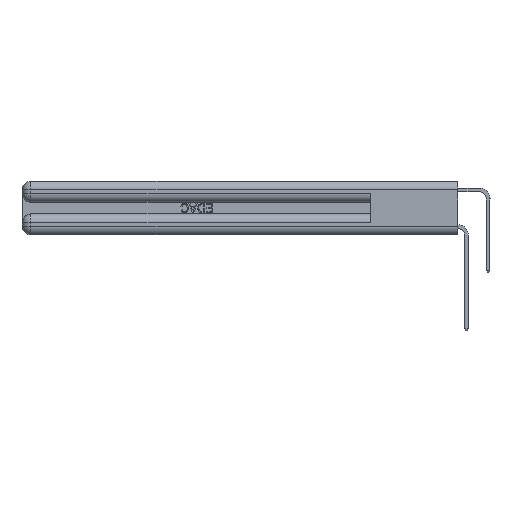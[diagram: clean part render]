
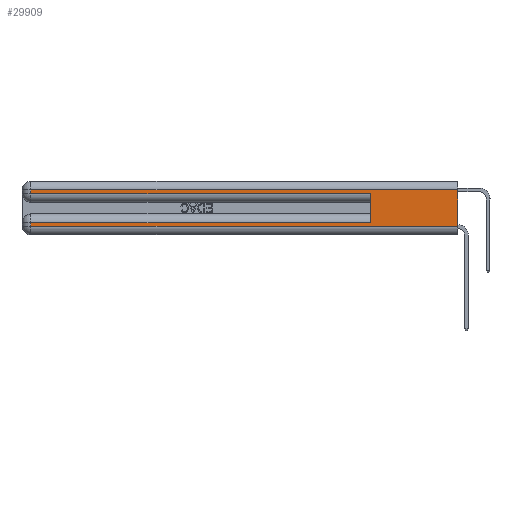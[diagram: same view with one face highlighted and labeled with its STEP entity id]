
A CAD part, left-side view. The second image highlights one B-rep face of the part: STEP entity #29909.
In plain terms, the highlighted planar face has unit normal (-1, 0, 0).
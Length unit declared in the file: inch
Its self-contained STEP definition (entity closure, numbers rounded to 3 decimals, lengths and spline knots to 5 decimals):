
#688 = CARTESIAN_POINT ( 'NONE',  ( 0., 0., 0.31 ) ) ;
#2216 = DIRECTION ( 'NONE',  ( 0., 0., -1. ) ) ;
#2385 = CARTESIAN_POINT ( 'NONE',  ( 0., 0.6, 0.285 ) ) ;
#2524 = EDGE_CURVE ( 'NONE', #15387, #31650, #4604, .T. ) ;
#3878 = CARTESIAN_POINT ( 'NONE',  ( 0., 0., 0.06 ) ) ;
#4311 = FACE_OUTER_BOUND ( 'NONE', #28286, .T. ) ;
#4604 = LINE ( 'NONE', #30196, #15029 ) ;
#4754 = DIRECTION ( 'NONE',  ( 1., 0., 0. ) ) ;
#4879 = CARTESIAN_POINT ( 'NONE',  ( 0., 0., 0.085 ) ) ;
#4961 = CARTESIAN_POINT ( 'NONE',  ( 0., 0.6, 0.145 ) ) ;
#4972 = DIRECTION ( 'NONE',  ( 0., -1., 0. ) ) ;
#5525 = LINE ( 'NONE', #33076, #29310 ) ;
#6470 = LINE ( 'NONE', #688, #27855 ) ;
#6865 = LINE ( 'NONE', #4879, #18047 ) ;
#7455 = DIRECTION ( 'NONE',  ( 0., 0., -1. ) ) ;
#8250 = EDGE_CURVE ( 'NONE', #22553, #27764, #6470, .T. ) ;
#8692 = VERTEX_POINT ( 'NONE', #15532 ) ;
#9332 = ORIENTED_EDGE ( 'NONE', *, *, #22059, .T. ) ;
#9527 = VECTOR ( 'NONE', #7455, 39.37008 ) ;
#10952 = ORIENTED_EDGE ( 'NONE', *, *, #20785, .F. ) ;
#11116 = LINE ( 'NONE', #4961, #17175 ) ;
#11144 = CARTESIAN_POINT ( 'NONE',  ( 0., 2.94, 0.31 ) ) ;
#13689 = CARTESIAN_POINT ( 'NONE',  ( 0., 2.94, 0.285 ) ) ;
#13787 = CARTESIAN_POINT ( 'NONE',  ( 0., 0., 0.06 ) ) ;
#13980 = CARTESIAN_POINT ( 'NONE',  ( 0., 0., 0.37 ) ) ;
#14259 = VERTEX_POINT ( 'NONE', #28304 ) ;
#14722 = LINE ( 'NONE', #20456, #9527 ) ;
#15029 = VECTOR ( 'NONE', #4972, 39.37008 ) ;
#15387 = VERTEX_POINT ( 'NONE', #13689 ) ;
#15532 = CARTESIAN_POINT ( 'NONE',  ( 0., 2.94, 0.06 ) ) ;
#16573 = LINE ( 'NONE', #13787, #28685 ) ;
#17175 = VECTOR ( 'NONE', #18098, 39.37008 ) ;
#17604 = ORIENTED_EDGE ( 'NONE', *, *, #8250, .T. ) ;
#17777 = CARTESIAN_POINT ( 'NONE',  ( 0., 0., 0.37 ) ) ;
#18047 = VECTOR ( 'NONE', #20168, 39.37008 ) ;
#18098 = DIRECTION ( 'NONE',  ( 0., 0., 1. ) ) ;
#18941 = DIRECTION ( 'NONE',  ( 0., 0., -1. ) ) ;
#19156 = CARTESIAN_POINT ( 'NONE',  ( 0., 0., 0.31 ) ) ;
#19185 = VERTEX_POINT ( 'NONE', #3878 ) ;
#19994 = AXIS2_PLACEMENT_3D ( 'NONE', #17777, #4754, #30559 ) ;
#20168 = DIRECTION ( 'NONE',  ( 0., 1., 0. ) ) ;
#20456 = CARTESIAN_POINT ( 'NONE',  ( 0., 2.94, 0.37 ) ) ;
#20785 = EDGE_CURVE ( 'NONE', #22553, #19185, #29424, .T. ) ;
#20949 = DIRECTION ( 'NONE',  ( 0., 1., 0. ) ) ;
#22059 = EDGE_CURVE ( 'NONE', #28037, #14259, #6865, .T. ) ;
#22553 = VERTEX_POINT ( 'NONE', #19156 ) ;
#23087 = PLANE ( 'NONE',  #19994 ) ;
#23167 = ORIENTED_EDGE ( 'NONE', *, *, #28883, .T. ) ;
#24087 = EDGE_CURVE ( 'NONE', #27764, #15387, #14722, .T. ) ;
#24133 = EDGE_CURVE ( 'NONE', #28037, #31650, #11116, .T. ) ;
#24204 = ORIENTED_EDGE ( 'NONE', *, *, #2524, .T. ) ;
#25109 = ORIENTED_EDGE ( 'NONE', *, *, #26220, .T. ) ;
#26220 = EDGE_CURVE ( 'NONE', #8692, #19185, #16573, .T. ) ;
#26471 = DIRECTION ( 'NONE',  ( 0., -1., 0. ) ) ;
#27083 = ORIENTED_EDGE ( 'NONE', *, *, #24133, .F. ) ;
#27510 = CARTESIAN_POINT ( 'NONE',  ( 0., 0.6, 0.085 ) ) ;
#27764 = VERTEX_POINT ( 'NONE', #11144 ) ;
#27855 = VECTOR ( 'NONE', #20949, 39.37008 ) ;
#28037 = VERTEX_POINT ( 'NONE', #27510 ) ;
#28286 = EDGE_LOOP ( 'NONE', ( #10952, #17604, #28562, #24204, #27083, #9332, #23167, #25109 ) ) ;
#28304 = CARTESIAN_POINT ( 'NONE',  ( 0., 2.94, 0.085 ) ) ;
#28562 = ORIENTED_EDGE ( 'NONE', *, *, #24087, .T. ) ;
#28685 = VECTOR ( 'NONE', #26471, 39.37008 ) ;
#28883 = EDGE_CURVE ( 'NONE', #14259, #8692, #5525, .T. ) ;
#29310 = VECTOR ( 'NONE', #2216, 39.37008 ) ;
#29424 = LINE ( 'NONE', #13980, #30257 ) ;
#29909 = ADVANCED_FACE ( 'NONE', ( #4311 ), #23087, .F. ) ;
#30196 = CARTESIAN_POINT ( 'NONE',  ( 0., 0., 0.285 ) ) ;
#30257 = VECTOR ( 'NONE', #18941, 39.37008 ) ;
#30559 = DIRECTION ( 'NONE',  ( 0., 0., -1. ) ) ;
#31650 = VERTEX_POINT ( 'NONE', #2385 ) ;
#33076 = CARTESIAN_POINT ( 'NONE',  ( 0., 2.94, 0.37 ) ) ;
